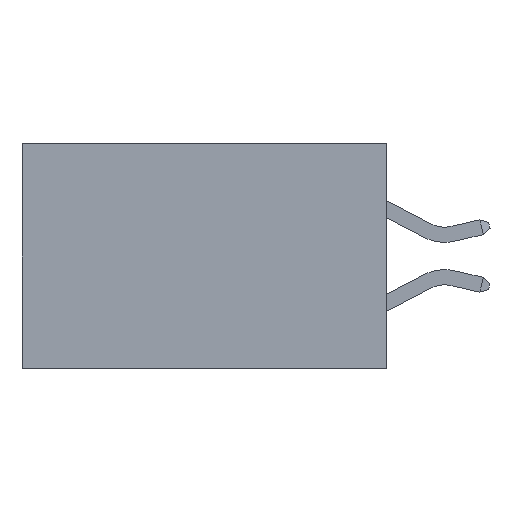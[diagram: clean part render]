
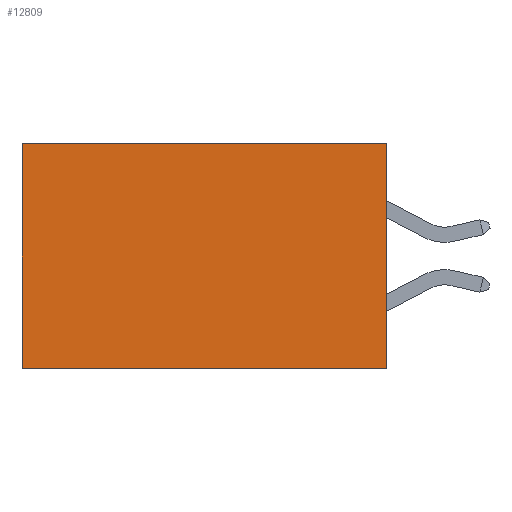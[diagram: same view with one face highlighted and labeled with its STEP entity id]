
A CAD part, left-side view. The second image highlights one B-rep face of the part: STEP entity #12809.
In plain terms, the highlighted planar face has unit normal (-1, 0, 0).
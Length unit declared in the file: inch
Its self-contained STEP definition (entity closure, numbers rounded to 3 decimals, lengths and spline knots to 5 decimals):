
#159 = VECTOR ( 'NONE', #15564, 39.37008 ) ;
#272 = EDGE_CURVE ( 'NONE', #10738, #15355, #9627, .T. ) ;
#274 = LINE ( 'NONE', #7540, #7215 ) ;
#342 = LINE ( 'NONE', #2527, #440 ) ;
#440 = VECTOR ( 'NONE', #7719, 39.37008 ) ;
#1092 = VERTEX_POINT ( 'NONE', #11049 ) ;
#1677 = DIRECTION ( 'NONE',  ( 0., 0., -1. ) ) ;
#2405 = AXIS2_PLACEMENT_3D ( 'NONE', #18396, #9174, #1677 ) ;
#2527 = CARTESIAN_POINT ( 'NONE',  ( 0.2615, 0., 0. ) ) ;
#2871 = CARTESIAN_POINT ( 'NONE',  ( 0.2615, 0., -0.37 ) ) ;
#3019 = ORIENTED_EDGE ( 'NONE', *, *, #14790, .F. ) ;
#3491 = FACE_OUTER_BOUND ( 'NONE', #22683, .T. ) ;
#7215 = VECTOR ( 'NONE', #15283, 39.37008 ) ;
#7489 = ORIENTED_EDGE ( 'NONE', *, *, #272, .F. ) ;
#7540 = CARTESIAN_POINT ( 'NONE',  ( 0.2615, 0.6, -0.37 ) ) ;
#7700 = DIRECTION ( 'NONE',  ( 0., 0., -1. ) ) ;
#7719 = DIRECTION ( 'NONE',  ( 0., 1., 0. ) ) ;
#9174 = DIRECTION ( 'NONE',  ( 1., 0., 0. ) ) ;
#9627 = LINE ( 'NONE', #15572, #16856 ) ;
#10357 = EDGE_CURVE ( 'NONE', #10738, #21529, #342, .T. ) ;
#10574 = ORIENTED_EDGE ( 'NONE', *, *, #19777, .T. ) ;
#10715 = ORIENTED_EDGE ( 'NONE', *, *, #10357, .T. ) ;
#10738 = VERTEX_POINT ( 'NONE', #20868 ) ;
#11049 = CARTESIAN_POINT ( 'NONE',  ( 0.2615, 0.6, -0.37 ) ) ;
#12809 = ADVANCED_FACE ( 'NONE', ( #3491 ), #18269, .F. ) ;
#14790 = EDGE_CURVE ( 'NONE', #15355, #1092, #19574, .T. ) ;
#14902 = CARTESIAN_POINT ( 'NONE',  ( 0.2615, 0.6, 0. ) ) ;
#15283 = DIRECTION ( 'NONE',  ( 0., 0., -1. ) ) ;
#15355 = VERTEX_POINT ( 'NONE', #2871 ) ;
#15564 = DIRECTION ( 'NONE',  ( 0., 1., 0. ) ) ;
#15572 = CARTESIAN_POINT ( 'NONE',  ( 0.2615, 0., -0.37 ) ) ;
#16856 = VECTOR ( 'NONE', #7700, 39.37008 ) ;
#17507 = CARTESIAN_POINT ( 'NONE',  ( 0.2615, 0., -0.37 ) ) ;
#18269 = PLANE ( 'NONE',  #2405 ) ;
#18396 = CARTESIAN_POINT ( 'NONE',  ( 0.2615, 0., -0.37 ) ) ;
#19574 = LINE ( 'NONE', #17507, #159 ) ;
#19777 = EDGE_CURVE ( 'NONE', #21529, #1092, #274, .T. ) ;
#20868 = CARTESIAN_POINT ( 'NONE',  ( 0.2615, 0., 0. ) ) ;
#21529 = VERTEX_POINT ( 'NONE', #14902 ) ;
#22683 = EDGE_LOOP ( 'NONE', ( #10574, #3019, #7489, #10715 ) ) ;
